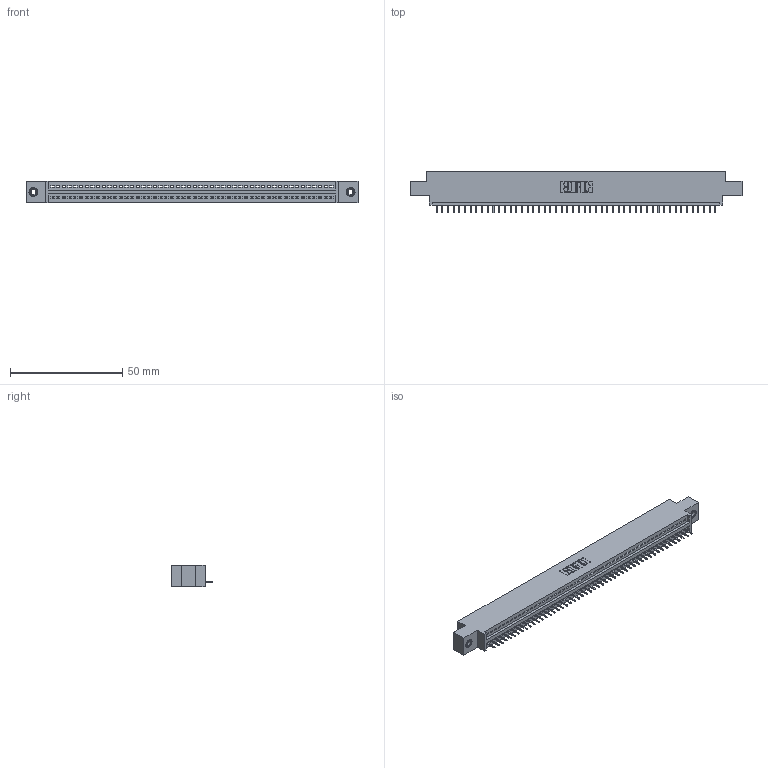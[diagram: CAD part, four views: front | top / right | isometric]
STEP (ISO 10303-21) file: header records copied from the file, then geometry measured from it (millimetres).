
FILE_DESCRIPTION (( 'STEP AP203' ), '1' );
FILE_NAME ('395-050-525-608.STEP', '2020-09-24T10:13:24', ( '' ), ( '' ), 'SwSTEP 2.0', 'SolidWorks 2020', '' );
FILE_SCHEMA (( 'CONFIG_CONTROL_DESIGN' ));
Length unit declared in the file: inch
Products named in the file (4): 395-050-525-608; 345-292-001_345-293-125; 345-250-001_345-250-003-102; 345 Part_0.170 Offset - 0.156 Dia-TI
Assembly tree (53 placements, depth 2):
  395-050-525-608
    345 Part_0.170 Offset - 0.156 Dia-TI
    345-292-001_345-293-125  x50
    345-250-001_345-250-003-102  x2
Bounding box: 148.21 x 18.72 x 9.4 mm (x, y, z)
Volume: 13818.5 mm3; surface area: 17937.2 mm2
Topology: 53 solids, 53 shells, 3290 faces, 9489 edges, 6118 vertices
Faces by surface type: plane 2416, cylinder 858, cone 12, torus 4
Entity records: 37946 total; most frequent: CARTESIAN_POINT 6553, ORIENTED_EDGE 6530, DIRECTION 5739, EDGE_CURVE 3265, LINE 2917, VECTOR 2917, VERTEX_POINT 2168, AXIS2_PLACEMENT_3D 1411
